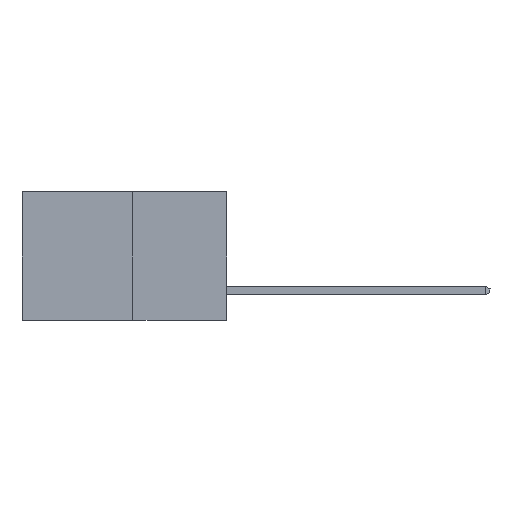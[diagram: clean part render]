
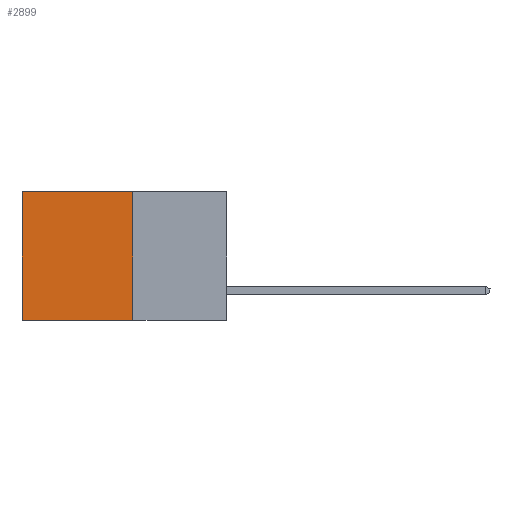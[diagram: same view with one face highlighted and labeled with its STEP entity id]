
A CAD part, left-side view. The second image highlights one B-rep face of the part: STEP entity #2899.
In plain terms, the highlighted planar face has unit normal (-1, 0, 0).
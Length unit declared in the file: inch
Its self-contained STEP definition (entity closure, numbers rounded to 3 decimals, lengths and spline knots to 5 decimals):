
#553 = VERTEX_POINT ( 'NONE', #10335 ) ;
#616 = DIRECTION ( 'NONE',  ( 0., 1., 0. ) ) ;
#1124 = CARTESIAN_POINT ( 'NONE',  ( 0.277, 0.27, -0.37 ) ) ;
#1198 = EDGE_CURVE ( 'NONE', #15848, #553, #14215, .T. ) ;
#1533 = DIRECTION ( 'NONE',  ( 0., 1., 0. ) ) ;
#1651 = LINE ( 'NONE', #13710, #11372 ) ;
#1806 = EDGE_CURVE ( 'NONE', #15561, #13815, #1651, .T. ) ;
#2221 = CARTESIAN_POINT ( 'NONE',  ( 0.277, 0.27, -0.37 ) ) ;
#2899 = ADVANCED_FACE ( 'NONE', ( #4117 ), #10947, .F. ) ;
#3794 = VECTOR ( 'NONE', #11553, 39.37008 ) ;
#4035 = CARTESIAN_POINT ( 'NONE',  ( 0.277, 0.59, 0. ) ) ;
#4117 = FACE_OUTER_BOUND ( 'NONE', #8774, .T. ) ;
#4534 = AXIS2_PLACEMENT_3D ( 'NONE', #2221, #11942, #11803 ) ;
#4555 = CARTESIAN_POINT ( 'NONE',  ( 0.277, 0.27, 0. ) ) ;
#4693 = CARTESIAN_POINT ( 'NONE',  ( 0.277, 0.27, 0. ) ) ;
#4735 = LINE ( 'NONE', #1124, #14776 ) ;
#4835 = EDGE_CURVE ( 'NONE', #553, #13815, #4735, .T. ) ;
#6408 = LINE ( 'NONE', #4555, #9535 ) ;
#7413 = CARTESIAN_POINT ( 'NONE',  ( 0.277, 0.27, -0.37 ) ) ;
#8774 = EDGE_LOOP ( 'NONE', ( #13763, #10749, #11543, #14971 ) ) ;
#9535 = VECTOR ( 'NONE', #616, 39.37008 ) ;
#10335 = CARTESIAN_POINT ( 'NONE',  ( 0.277, 0.27, -0.37 ) ) ;
#10749 = ORIENTED_EDGE ( 'NONE', *, *, #4835, .F. ) ;
#10947 = PLANE ( 'NONE',  #4534 ) ;
#11372 = VECTOR ( 'NONE', #12569, 39.37008 ) ;
#11543 = ORIENTED_EDGE ( 'NONE', *, *, #1198, .F. ) ;
#11553 = DIRECTION ( 'NONE',  ( 0., 0., -1. ) ) ;
#11803 = DIRECTION ( 'NONE',  ( 0., 0., -1. ) ) ;
#11942 = DIRECTION ( 'NONE',  ( 1., 0., 0. ) ) ;
#12569 = DIRECTION ( 'NONE',  ( 0., 0., -1. ) ) ;
#12863 = EDGE_CURVE ( 'NONE', #15848, #15561, #6408, .T. ) ;
#13710 = CARTESIAN_POINT ( 'NONE',  ( 0.277, 0.59, -0.37 ) ) ;
#13763 = ORIENTED_EDGE ( 'NONE', *, *, #1806, .T. ) ;
#13815 = VERTEX_POINT ( 'NONE', #14317 ) ;
#14215 = LINE ( 'NONE', #7413, #3794 ) ;
#14317 = CARTESIAN_POINT ( 'NONE',  ( 0.277, 0.59, -0.37 ) ) ;
#14776 = VECTOR ( 'NONE', #1533, 39.37008 ) ;
#14971 = ORIENTED_EDGE ( 'NONE', *, *, #12863, .T. ) ;
#15561 = VERTEX_POINT ( 'NONE', #4035 ) ;
#15848 = VERTEX_POINT ( 'NONE', #4693 ) ;
